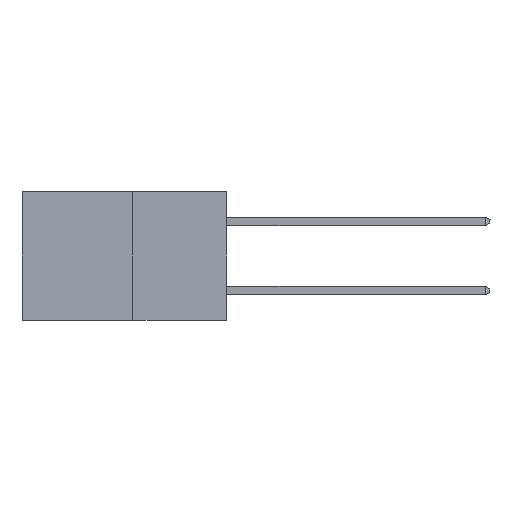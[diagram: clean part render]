
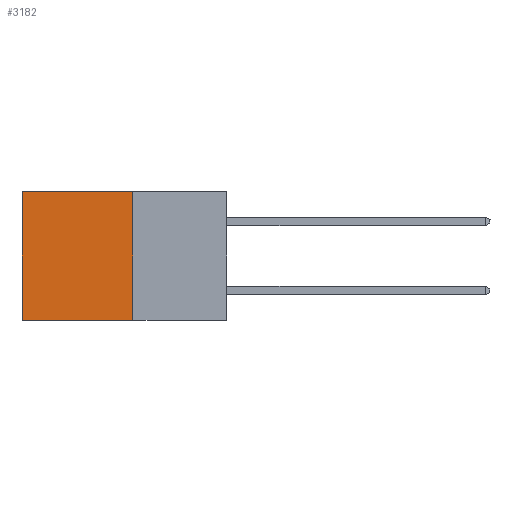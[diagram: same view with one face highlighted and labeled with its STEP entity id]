
A CAD part, left-side view. The second image highlights one B-rep face of the part: STEP entity #3182.
In plain terms, the highlighted planar face has unit normal (-1, 0, 0).
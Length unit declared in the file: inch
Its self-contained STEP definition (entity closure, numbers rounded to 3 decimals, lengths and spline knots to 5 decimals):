
#567 = CARTESIAN_POINT ( 'NONE',  ( 0.277, 0.27, -0.37 ) ) ;
#635 = ORIENTED_EDGE ( 'NONE', *, *, #7330, .T. ) ;
#1333 = LINE ( 'NONE', #567, #15731 ) ;
#1451 = DIRECTION ( 'NONE',  ( 1., 0., 0. ) ) ;
#1582 = CARTESIAN_POINT ( 'NONE',  ( 0.277, 0.27, -0.37 ) ) ;
#2065 = DIRECTION ( 'NONE',  ( 0., 0., -1. ) ) ;
#2226 = DIRECTION ( 'NONE',  ( 0., 0., -1. ) ) ;
#3094 = ORIENTED_EDGE ( 'NONE', *, *, #13877, .F. ) ;
#3182 = ADVANCED_FACE ( 'NONE', ( #3366 ), #14862, .F. ) ;
#3366 = FACE_OUTER_BOUND ( 'NONE', #12298, .T. ) ;
#3540 = ORIENTED_EDGE ( 'NONE', *, *, #4783, .F. ) ;
#3889 = VECTOR ( 'NONE', #8782, 39.37008 ) ;
#4783 = EDGE_CURVE ( 'NONE', #6716, #8646, #5939, .T. ) ;
#4845 = DIRECTION ( 'NONE',  ( 0., 1., 0. ) ) ;
#5939 = LINE ( 'NONE', #9401, #16562 ) ;
#6716 = VERTEX_POINT ( 'NONE', #12711 ) ;
#7146 = VERTEX_POINT ( 'NONE', #12506 ) ;
#7330 = EDGE_CURVE ( 'NONE', #6716, #7146, #11234, .T. ) ;
#8273 = CARTESIAN_POINT ( 'NONE',  ( 0.277, 0.59, -0.37 ) ) ;
#8646 = VERTEX_POINT ( 'NONE', #12286 ) ;
#8782 = DIRECTION ( 'NONE',  ( 0., 1., 0. ) ) ;
#9216 = DIRECTION ( 'NONE',  ( 0., 0., -1. ) ) ;
#9235 = VERTEX_POINT ( 'NONE', #8273 ) ;
#9363 = CARTESIAN_POINT ( 'NONE',  ( 0.277, 0.27, 0. ) ) ;
#9401 = CARTESIAN_POINT ( 'NONE',  ( 0.277, 0.27, -0.37 ) ) ;
#10051 = ORIENTED_EDGE ( 'NONE', *, *, #14470, .T. ) ;
#10281 = VECTOR ( 'NONE', #2226, 39.37008 ) ;
#11234 = LINE ( 'NONE', #9363, #3889 ) ;
#12286 = CARTESIAN_POINT ( 'NONE',  ( 0.277, 0.27, -0.37 ) ) ;
#12298 = EDGE_LOOP ( 'NONE', ( #10051, #3094, #3540, #635 ) ) ;
#12506 = CARTESIAN_POINT ( 'NONE',  ( 0.277, 0.59, 0. ) ) ;
#12711 = CARTESIAN_POINT ( 'NONE',  ( 0.277, 0.27, 0. ) ) ;
#13533 = LINE ( 'NONE', #17487, #10281 ) ;
#13877 = EDGE_CURVE ( 'NONE', #8646, #9235, #1333, .T. ) ;
#14470 = EDGE_CURVE ( 'NONE', #7146, #9235, #13533, .T. ) ;
#14862 = PLANE ( 'NONE',  #15373 ) ;
#15373 = AXIS2_PLACEMENT_3D ( 'NONE', #1582, #1451, #2065 ) ;
#15731 = VECTOR ( 'NONE', #4845, 39.37008 ) ;
#16562 = VECTOR ( 'NONE', #9216, 39.37008 ) ;
#17487 = CARTESIAN_POINT ( 'NONE',  ( 0.277, 0.59, -0.37 ) ) ;
